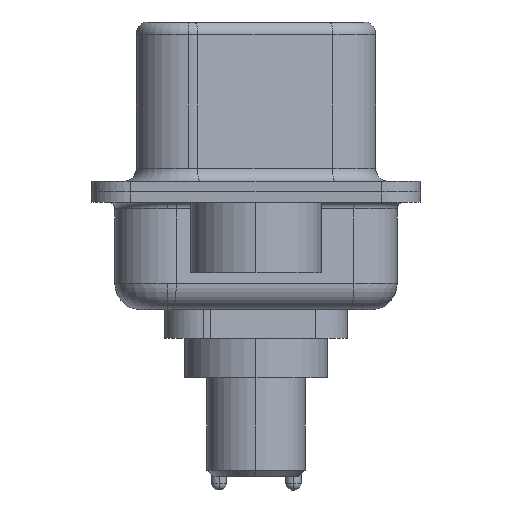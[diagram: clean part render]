
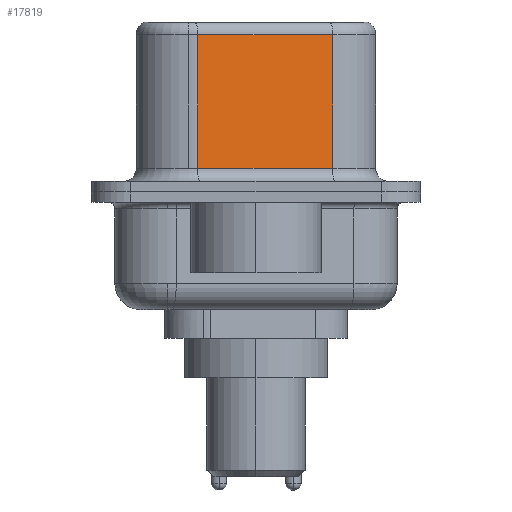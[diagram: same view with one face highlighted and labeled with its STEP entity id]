
A CAD part, left-side view. The second image highlights one B-rep face of the part: STEP entity #17819.
In plain terms, the highlighted planar face has unit normal (-0.985, -0.174, 0).
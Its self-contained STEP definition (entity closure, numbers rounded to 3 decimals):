
#684 = VERTEX_POINT ( 'NONE', #16660 ) ;
#1447 = CARTESIAN_POINT ( 'NONE',  ( 4.585, -2.927, 6.52 ) ) ;
#1643 = VECTOR ( 'NONE', #9968, 1000. ) ;
#2361 = PLANE ( 'NONE',  #12885 ) ;
#2801 = LINE ( 'NONE', #4734, #10243 ) ;
#3764 = EDGE_CURVE ( 'NONE', #684, #13523, #5392, .T. ) ;
#4171 = VERTEX_POINT ( 'NONE', #17324 ) ;
#4473 = CARTESIAN_POINT ( 'NONE',  ( 4.585, -2.927, 0.9 ) ) ;
#4734 = CARTESIAN_POINT ( 'NONE',  ( 4.585, -2.927, 6.02 ) ) ;
#5213 = DIRECTION ( 'NONE',  ( -0.174, 0.985, 0. ) ) ;
#5392 = LINE ( 'NONE', #6879, #1643 ) ;
#6751 = LINE ( 'NONE', #1447, #12872 ) ;
#6879 = CARTESIAN_POINT ( 'NONE',  ( 3.675, 2.233, 6.52 ) ) ;
#7122 = EDGE_CURVE ( 'NONE', #13523, #10635, #15465, .T. ) ;
#7359 = EDGE_LOOP ( 'NONE', ( #10076, #10155, #14836, #12656 ) ) ;
#7928 = VECTOR ( 'NONE', #17165, 1000. ) ;
#7937 = CARTESIAN_POINT ( 'NONE',  ( 3.675, 2.233, 0.9 ) ) ;
#7969 = CARTESIAN_POINT ( 'NONE',  ( 4.585, -2.927, 6.52 ) ) ;
#8834 = EDGE_CURVE ( 'NONE', #4171, #684, #2801, .T. ) ;
#9704 = FACE_OUTER_BOUND ( 'NONE', #7359, .T. ) ;
#9821 = DIRECTION ( 'NONE',  ( 0., 0., -1. ) ) ;
#9968 = DIRECTION ( 'NONE',  ( 0., 0., -1. ) ) ;
#10076 = ORIENTED_EDGE ( 'NONE', *, *, #15638, .F. ) ;
#10155 = ORIENTED_EDGE ( 'NONE', *, *, #8834, .T. ) ;
#10243 = VECTOR ( 'NONE', #14587, 1000. ) ;
#10635 = VERTEX_POINT ( 'NONE', #13879 ) ;
#12656 = ORIENTED_EDGE ( 'NONE', *, *, #7122, .T. ) ;
#12872 = VECTOR ( 'NONE', #9821, 1000. ) ;
#12885 = AXIS2_PLACEMENT_3D ( 'NONE', #7969, #13624, #5213 ) ;
#13523 = VERTEX_POINT ( 'NONE', #7937 ) ;
#13624 = DIRECTION ( 'NONE',  ( 0.985, 0.174, 0. ) ) ;
#13879 = CARTESIAN_POINT ( 'NONE',  ( 4.585, -2.927, 0.9 ) ) ;
#14587 = DIRECTION ( 'NONE',  ( -0.174, 0.985, 0. ) ) ;
#14836 = ORIENTED_EDGE ( 'NONE', *, *, #3764, .T. ) ;
#15465 = LINE ( 'NONE', #4473, #7928 ) ;
#15638 = EDGE_CURVE ( 'NONE', #4171, #10635, #6751, .T. ) ;
#16660 = CARTESIAN_POINT ( 'NONE',  ( 3.675, 2.233, 6.02 ) ) ;
#17165 = DIRECTION ( 'NONE',  ( 0.174, -0.985, 0. ) ) ;
#17324 = CARTESIAN_POINT ( 'NONE',  ( 4.585, -2.927, 6.02 ) ) ;
#17819 = ADVANCED_FACE ( 'NONE', ( #9704 ), #2361, .F. ) ;
